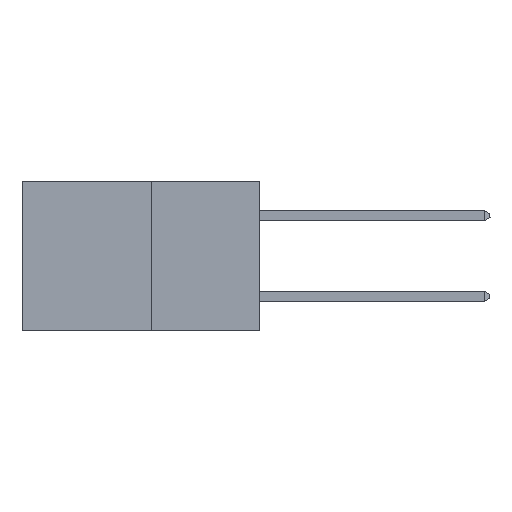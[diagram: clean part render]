
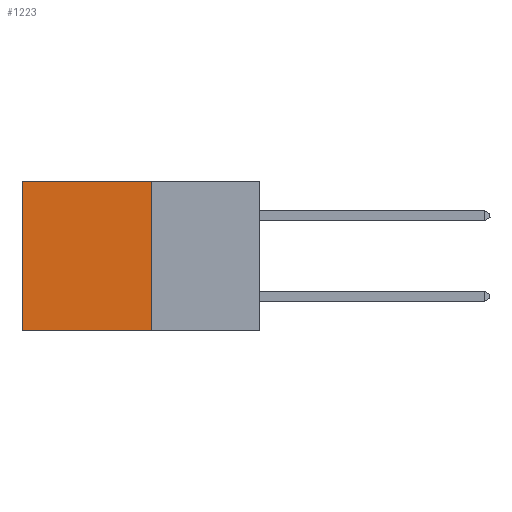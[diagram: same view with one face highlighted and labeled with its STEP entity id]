
A CAD part, left-side view. The second image highlights one B-rep face of the part: STEP entity #1223.
In plain terms, the highlighted planar face has unit normal (-1, 0, 0).
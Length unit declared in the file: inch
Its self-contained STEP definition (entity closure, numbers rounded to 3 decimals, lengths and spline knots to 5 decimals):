
#37 = VERTEX_POINT ( 'NONE', #5504 ) ;
#373 = CARTESIAN_POINT ( 'NONE',  ( 0.277, 0.59, -0.37 ) ) ;
#1217 = VECTOR ( 'NONE', #8769, 39.37008 ) ;
#1223 = ADVANCED_FACE ( 'NONE', ( #4348 ), #4117, .F. ) ;
#1625 = EDGE_CURVE ( 'NONE', #37, #4814, #7969, .T. ) ;
#2576 = ORIENTED_EDGE ( 'NONE', *, *, #4646, .F. ) ;
#2647 = VECTOR ( 'NONE', #6707, 39.37008 ) ;
#2798 = DIRECTION ( 'NONE',  ( 0., 0., -1. ) ) ;
#2849 = EDGE_LOOP ( 'NONE', ( #4052, #6405, #2576, #3232 ) ) ;
#3009 = CARTESIAN_POINT ( 'NONE',  ( 0.277, 0.27, 0. ) ) ;
#3098 = CARTESIAN_POINT ( 'NONE',  ( 0.277, 0.27, 0. ) ) ;
#3183 = LINE ( 'NONE', #3677, #8389 ) ;
#3232 = ORIENTED_EDGE ( 'NONE', *, *, #6798, .T. ) ;
#3677 = CARTESIAN_POINT ( 'NONE',  ( 0.277, 0.27, -0.37 ) ) ;
#4052 = ORIENTED_EDGE ( 'NONE', *, *, #7636, .T. ) ;
#4117 = PLANE ( 'NONE',  #7568 ) ;
#4127 = DIRECTION ( 'NONE',  ( 1., 0., 0. ) ) ;
#4220 = CARTESIAN_POINT ( 'NONE',  ( 0.277, 0.59, -0.37 ) ) ;
#4306 = CARTESIAN_POINT ( 'NONE',  ( 0.277, 0.27, -0.37 ) ) ;
#4348 = FACE_OUTER_BOUND ( 'NONE', #2849, .T. ) ;
#4646 = EDGE_CURVE ( 'NONE', #7196, #37, #3183, .T. ) ;
#4780 = LINE ( 'NONE', #373, #6202 ) ;
#4814 = VERTEX_POINT ( 'NONE', #4220 ) ;
#5284 = VERTEX_POINT ( 'NONE', #7305 ) ;
#5504 = CARTESIAN_POINT ( 'NONE',  ( 0.277, 0.27, -0.37 ) ) ;
#5640 = DIRECTION ( 'NONE',  ( 0., 0., -1. ) ) ;
#6202 = VECTOR ( 'NONE', #2798, 39.37008 ) ;
#6394 = CARTESIAN_POINT ( 'NONE',  ( 0.277, 0.27, -0.37 ) ) ;
#6405 = ORIENTED_EDGE ( 'NONE', *, *, #1625, .F. ) ;
#6707 = DIRECTION ( 'NONE',  ( 0., 1., 0. ) ) ;
#6798 = EDGE_CURVE ( 'NONE', #7196, #5284, #6988, .T. ) ;
#6988 = LINE ( 'NONE', #3009, #1217 ) ;
#7196 = VERTEX_POINT ( 'NONE', #3098 ) ;
#7305 = CARTESIAN_POINT ( 'NONE',  ( 0.277, 0.59, 0. ) ) ;
#7568 = AXIS2_PLACEMENT_3D ( 'NONE', #4306, #4127, #7761 ) ;
#7636 = EDGE_CURVE ( 'NONE', #5284, #4814, #4780, .T. ) ;
#7761 = DIRECTION ( 'NONE',  ( 0., 0., -1. ) ) ;
#7969 = LINE ( 'NONE', #6394, #2647 ) ;
#8389 = VECTOR ( 'NONE', #5640, 39.37008 ) ;
#8769 = DIRECTION ( 'NONE',  ( 0., 1., 0. ) ) ;
